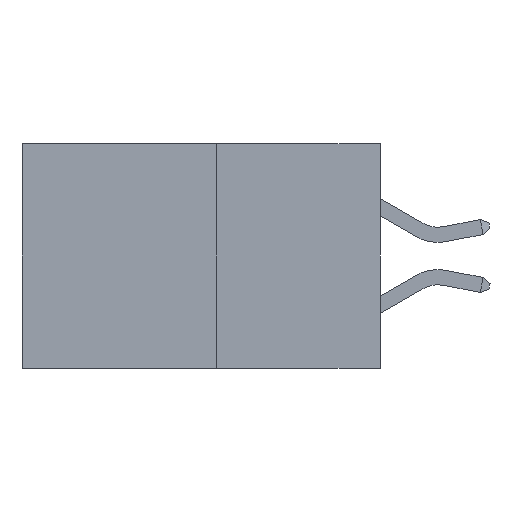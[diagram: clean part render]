
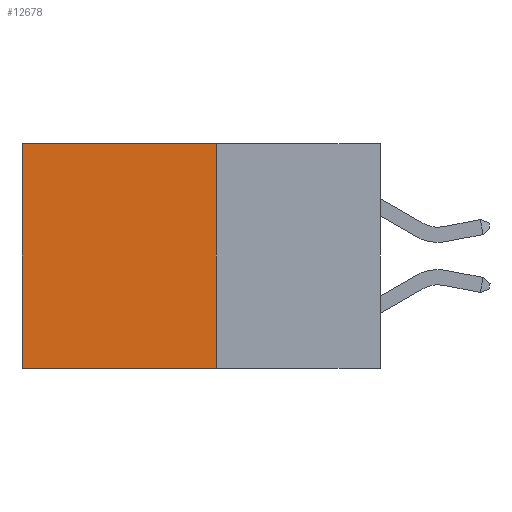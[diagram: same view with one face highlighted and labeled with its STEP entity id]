
A CAD part, left-side view. The second image highlights one B-rep face of the part: STEP entity #12678.
In plain terms, the highlighted planar face has unit normal (-1, 0, 0).
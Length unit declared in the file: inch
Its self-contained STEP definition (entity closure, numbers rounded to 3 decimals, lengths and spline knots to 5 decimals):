
#1054 = CARTESIAN_POINT ( 'NONE',  ( 0.277, 0.27, 0. ) ) ;
#1179 = LINE ( 'NONE', #7965, #3621 ) ;
#1228 = DIRECTION ( 'NONE',  ( 0., 0., -1. ) ) ;
#1255 = LINE ( 'NONE', #1335, #6960 ) ;
#1335 = CARTESIAN_POINT ( 'NONE',  ( 0.277, 0.59, -0.37 ) ) ;
#1500 = CARTESIAN_POINT ( 'NONE',  ( 0.277, 0.59, -0.37 ) ) ;
#1933 = EDGE_CURVE ( 'NONE', #9443, #12043, #7988, .T. ) ;
#1994 = DIRECTION ( 'NONE',  ( 0., 0., -1. ) ) ;
#2468 = DIRECTION ( 'NONE',  ( 0., 1., 0. ) ) ;
#3331 = DIRECTION ( 'NONE',  ( 1., 0., 0. ) ) ;
#3621 = VECTOR ( 'NONE', #5808, 39.37008 ) ;
#3657 = CARTESIAN_POINT ( 'NONE',  ( 0.277, 0.27, -0.37 ) ) ;
#4429 = FACE_OUTER_BOUND ( 'NONE', #5112, .T. ) ;
#5112 = EDGE_LOOP ( 'NONE', ( #6109, #8960, #12195, #6785 ) ) ;
#5808 = DIRECTION ( 'NONE',  ( 0., 1., 0. ) ) ;
#6109 = ORIENTED_EDGE ( 'NONE', *, *, #6697, .T. ) ;
#6697 = EDGE_CURVE ( 'NONE', #13880, #12043, #1255, .T. ) ;
#6785 = ORIENTED_EDGE ( 'NONE', *, *, #9366, .T. ) ;
#6960 = VECTOR ( 'NONE', #1228, 39.37008 ) ;
#7676 = VECTOR ( 'NONE', #2468, 39.37008 ) ;
#7965 = CARTESIAN_POINT ( 'NONE',  ( 0.277, 0.27, 0. ) ) ;
#7988 = LINE ( 'NONE', #10449, #7676 ) ;
#8014 = LINE ( 'NONE', #8665, #10937 ) ;
#8334 = AXIS2_PLACEMENT_3D ( 'NONE', #8779, #3331, #11024 ) ;
#8378 = VERTEX_POINT ( 'NONE', #1054 ) ;
#8665 = CARTESIAN_POINT ( 'NONE',  ( 0.277, 0.27, -0.37 ) ) ;
#8727 = PLANE ( 'NONE',  #8334 ) ;
#8779 = CARTESIAN_POINT ( 'NONE',  ( 0.277, 0.27, -0.37 ) ) ;
#8960 = ORIENTED_EDGE ( 'NONE', *, *, #1933, .F. ) ;
#9366 = EDGE_CURVE ( 'NONE', #8378, #13880, #1179, .T. ) ;
#9443 = VERTEX_POINT ( 'NONE', #3657 ) ;
#10381 = CARTESIAN_POINT ( 'NONE',  ( 0.277, 0.59, 0. ) ) ;
#10449 = CARTESIAN_POINT ( 'NONE',  ( 0.277, 0.27, -0.37 ) ) ;
#10937 = VECTOR ( 'NONE', #1994, 39.37008 ) ;
#11024 = DIRECTION ( 'NONE',  ( 0., 0., -1. ) ) ;
#11453 = EDGE_CURVE ( 'NONE', #8378, #9443, #8014, .T. ) ;
#12043 = VERTEX_POINT ( 'NONE', #1500 ) ;
#12195 = ORIENTED_EDGE ( 'NONE', *, *, #11453, .F. ) ;
#12678 = ADVANCED_FACE ( 'NONE', ( #4429 ), #8727, .F. ) ;
#13880 = VERTEX_POINT ( 'NONE', #10381 ) ;
